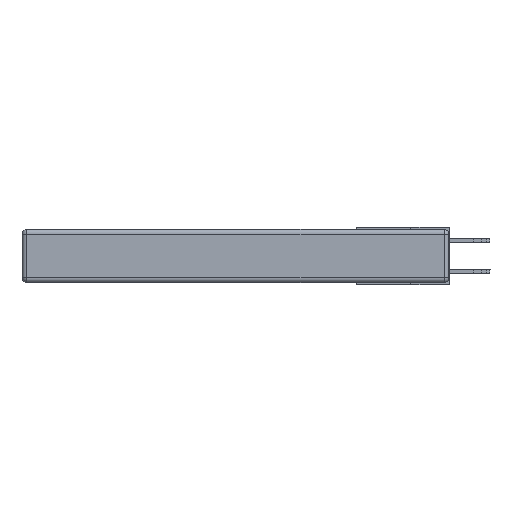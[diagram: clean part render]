
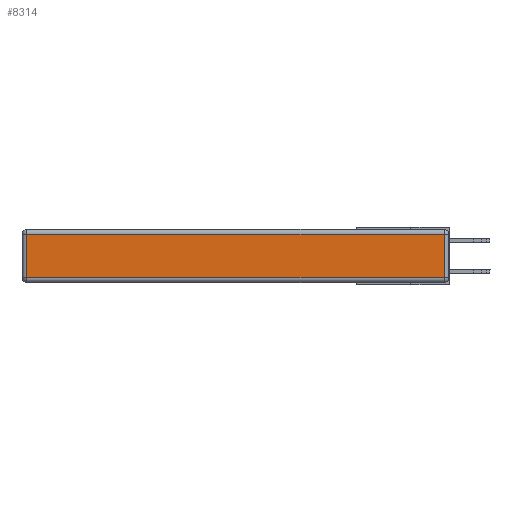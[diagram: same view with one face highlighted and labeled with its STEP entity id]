
A CAD part, left-side view. The second image highlights one B-rep face of the part: STEP entity #8314.
In plain terms, the highlighted planar face has unit normal (-1, 0, 0).
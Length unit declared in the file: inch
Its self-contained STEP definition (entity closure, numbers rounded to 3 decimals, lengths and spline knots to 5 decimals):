
#174 = EDGE_LOOP ( 'NONE', ( #2255, #12857, #2327, #3547 ) ) ;
#653 = CARTESIAN_POINT ( 'NONE',  ( 0., 2.72, -0.313 ) ) ;
#1049 = DIRECTION ( 'NONE',  ( 0., 1., 0. ) ) ;
#1739 = VERTEX_POINT ( 'NONE', #13231 ) ;
#1897 = DIRECTION ( 'NONE',  ( 0., 0., 1. ) ) ;
#2255 = ORIENTED_EDGE ( 'NONE', *, *, #12787, .T. ) ;
#2327 = ORIENTED_EDGE ( 'NONE', *, *, #4354, .T. ) ;
#3188 = CARTESIAN_POINT ( 'NONE',  ( 0., 0., -0.343 ) ) ;
#3547 = ORIENTED_EDGE ( 'NONE', *, *, #11789, .T. ) ;
#3566 = LINE ( 'NONE', #16372, #5929 ) ;
#4354 = EDGE_CURVE ( 'NONE', #1739, #13858, #3566, .T. ) ;
#4399 = DIRECTION ( 'NONE',  ( -1., 0., 0. ) ) ;
#4899 = CARTESIAN_POINT ( 'NONE',  ( 0., 2.72, -0.343 ) ) ;
#5133 = VERTEX_POINT ( 'NONE', #13251 ) ;
#5303 = DIRECTION ( 'NONE',  ( 0., 0., 1. ) ) ;
#5929 = VECTOR ( 'NONE', #1049, 39.37008 ) ;
#6250 = DIRECTION ( 'NONE',  ( 0., -1., 0. ) ) ;
#7148 = CARTESIAN_POINT ( 'NONE',  ( 0., 2.72, -0.03 ) ) ;
#8314 = ADVANCED_FACE ( 'NONE', ( #13638 ), #13370, .T. ) ;
#8876 = CARTESIAN_POINT ( 'NONE',  ( 0., 0., -0.313 ) ) ;
#10079 = DIRECTION ( 'NONE',  ( 0., 0., -1. ) ) ;
#10093 = VECTOR ( 'NONE', #10079, 39.37008 ) ;
#10715 = EDGE_CURVE ( 'NONE', #5133, #1739, #14590, .T. ) ;
#11070 = VECTOR ( 'NONE', #6250, 39.37008 ) ;
#11487 = LINE ( 'NONE', #8876, #11070 ) ;
#11517 = LINE ( 'NONE', #4899, #10093 ) ;
#11789 = EDGE_CURVE ( 'NONE', #13858, #15697, #11517, .T. ) ;
#12787 = EDGE_CURVE ( 'NONE', #15697, #5133, #11487, .T. ) ;
#12857 = ORIENTED_EDGE ( 'NONE', *, *, #10715, .T. ) ;
#13231 = CARTESIAN_POINT ( 'NONE',  ( 0., 0.03, -0.03 ) ) ;
#13251 = CARTESIAN_POINT ( 'NONE',  ( 0., 0.03, -0.313 ) ) ;
#13370 = PLANE ( 'NONE',  #14390 ) ;
#13638 = FACE_OUTER_BOUND ( 'NONE', #174, .T. ) ;
#13858 = VERTEX_POINT ( 'NONE', #7148 ) ;
#14390 = AXIS2_PLACEMENT_3D ( 'NONE', #3188, #4399, #1897 ) ;
#14454 = CARTESIAN_POINT ( 'NONE',  ( 0., 0.03, -0.343 ) ) ;
#14590 = LINE ( 'NONE', #14454, #15206 ) ;
#15206 = VECTOR ( 'NONE', #5303, 39.37008 ) ;
#15697 = VERTEX_POINT ( 'NONE', #653 ) ;
#16372 = CARTESIAN_POINT ( 'NONE',  ( 0., 2.75, -0.03 ) ) ;
